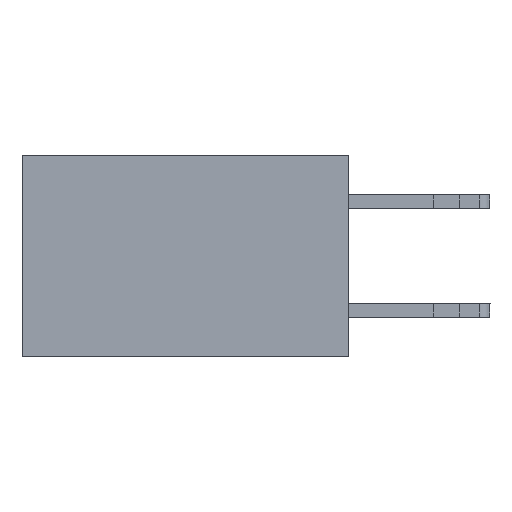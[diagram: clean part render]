
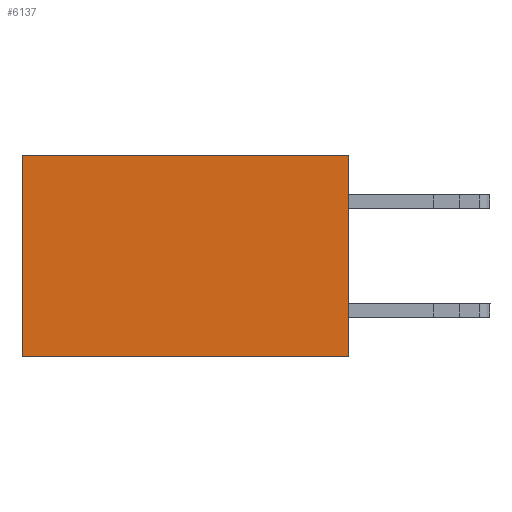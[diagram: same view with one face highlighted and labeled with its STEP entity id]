
A CAD part, left-side view. The second image highlights one B-rep face of the part: STEP entity #6137.
In plain terms, the highlighted planar face has unit normal (-1, 0, 0).
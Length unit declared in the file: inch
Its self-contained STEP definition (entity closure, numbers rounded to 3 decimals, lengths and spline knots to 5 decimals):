
#442 = CARTESIAN_POINT ( 'NONE',  ( 0.298, 0.6, 0. ) ) ;
#562 = LINE ( 'NONE', #3742, #15569 ) ;
#870 = EDGE_CURVE ( 'NONE', #15479, #17423, #562, .T. ) ;
#951 = CARTESIAN_POINT ( 'NONE',  ( 0.298, 0., -0.37 ) ) ;
#1102 = DIRECTION ( 'NONE',  ( 0., 1., 0. ) ) ;
#1434 = AXIS2_PLACEMENT_3D ( 'NONE', #15602, #10207, #1878 ) ;
#1878 = DIRECTION ( 'NONE',  ( 0., 0., -1. ) ) ;
#2012 = ORIENTED_EDGE ( 'NONE', *, *, #12521, .F. ) ;
#2423 = DIRECTION ( 'NONE',  ( 0., 1., 0. ) ) ;
#3742 = CARTESIAN_POINT ( 'NONE',  ( 0.298, 0., 0. ) ) ;
#4141 = EDGE_LOOP ( 'NONE', ( #14117, #2012, #7243, #13072 ) ) ;
#4901 = CARTESIAN_POINT ( 'NONE',  ( 0.298, 0.6, -0.37 ) ) ;
#5593 = FACE_OUTER_BOUND ( 'NONE', #4141, .T. ) ;
#6137 = ADVANCED_FACE ( 'NONE', ( #5593 ), #17049, .F. ) ;
#6221 = VERTEX_POINT ( 'NONE', #4901 ) ;
#6762 = CARTESIAN_POINT ( 'NONE',  ( 0.298, 0., -0.37 ) ) ;
#6859 = CARTESIAN_POINT ( 'NONE',  ( 0.298, 0., 0. ) ) ;
#6907 = DIRECTION ( 'NONE',  ( 0., 0., -1. ) ) ;
#7243 = ORIENTED_EDGE ( 'NONE', *, *, #16606, .F. ) ;
#8766 = CARTESIAN_POINT ( 'NONE',  ( 0.298, 0., 0. ) ) ;
#8819 = VECTOR ( 'NONE', #6907, 39.37008 ) ;
#10207 = DIRECTION ( 'NONE',  ( 1., 0., 0. ) ) ;
#11014 = VECTOR ( 'NONE', #12865, 39.37008 ) ;
#11240 = CARTESIAN_POINT ( 'NONE',  ( 0.298, 0.6, 0. ) ) ;
#11962 = VECTOR ( 'NONE', #2423, 39.37008 ) ;
#12521 = EDGE_CURVE ( 'NONE', #17312, #6221, #17578, .T. ) ;
#12865 = DIRECTION ( 'NONE',  ( 0., 0., -1. ) ) ;
#13072 = ORIENTED_EDGE ( 'NONE', *, *, #870, .T. ) ;
#14117 = ORIENTED_EDGE ( 'NONE', *, *, #16285, .T. ) ;
#14503 = LINE ( 'NONE', #442, #11014 ) ;
#15479 = VERTEX_POINT ( 'NONE', #6859 ) ;
#15569 = VECTOR ( 'NONE', #1102, 39.37008 ) ;
#15602 = CARTESIAN_POINT ( 'NONE',  ( 0.298, 0., 0. ) ) ;
#16200 = LINE ( 'NONE', #8766, #8819 ) ;
#16285 = EDGE_CURVE ( 'NONE', #17423, #6221, #14503, .T. ) ;
#16606 = EDGE_CURVE ( 'NONE', #15479, #17312, #16200, .T. ) ;
#17049 = PLANE ( 'NONE',  #1434 ) ;
#17312 = VERTEX_POINT ( 'NONE', #951 ) ;
#17423 = VERTEX_POINT ( 'NONE', #11240 ) ;
#17578 = LINE ( 'NONE', #6762, #11962 ) ;
